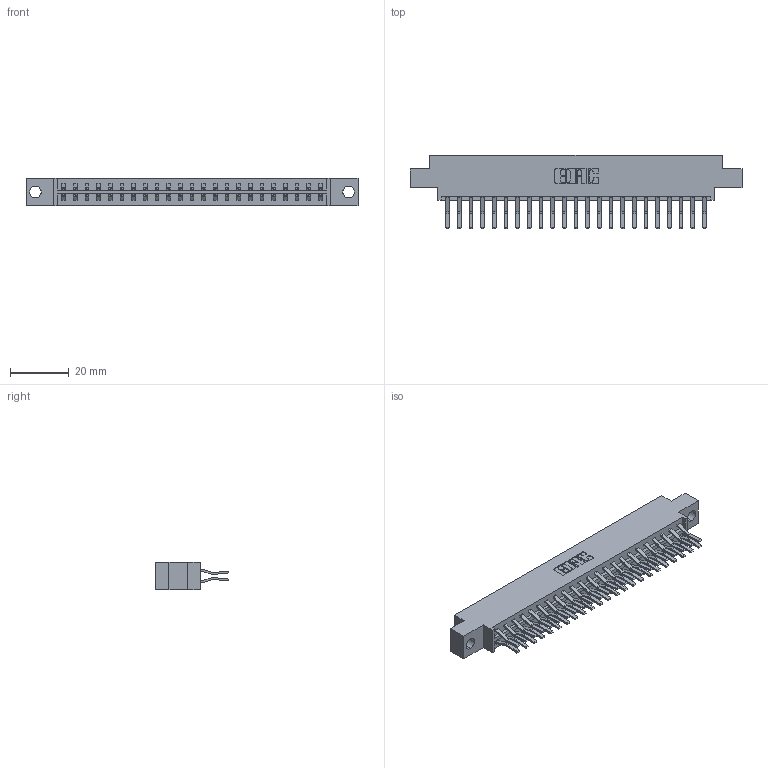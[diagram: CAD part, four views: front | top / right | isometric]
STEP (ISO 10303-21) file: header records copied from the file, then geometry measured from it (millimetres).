
FILE_DESCRIPTION (( 'STEP AP203' ), '1' );
FILE_NAME ('833-046-560-804.STEP', '2020-06-04T15:14:51', ( '' ), ( '' ), 'SwSTEP 2.0', 'SolidWorks 2020', '' );
FILE_SCHEMA (( 'CONFIG_CONTROL_DESIGN' ));
Length unit declared in the file: inch
Products named in the file (3): 833-046-560-804; 833 Part_Offset - .156 Dia - TH; 345-292-001_560 Tail
Assembly tree (47 placements, depth 2):
  833-046-560-804
    833 Part_Offset - .156 Dia - TH
    345-292-001_560 Tail  x46
Bounding box: 112.67 x 24.78 x 9.4 mm (x, y, z)
Volume: 11311.6 mm3; surface area: 14049.3 mm2
Topology: 47 solids, 47 shells, 2602 faces, 7729 edges, 5090 vertices
Faces by surface type: plane 1730, cylinder 872
Entity records: 17477 total; most frequent: CARTESIAN_POINT 2922, ORIENTED_EDGE 2858, DIRECTION 2533, EDGE_CURVE 1429, LINE 1297, VECTOR 1297, VERTEX_POINT 950, AXIS2_PLACEMENT_3D 618
